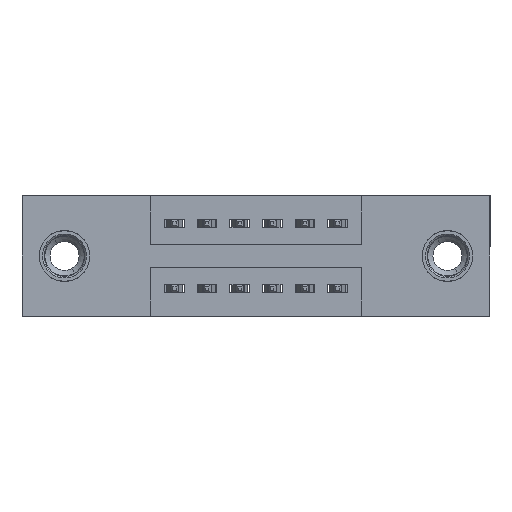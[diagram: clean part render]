
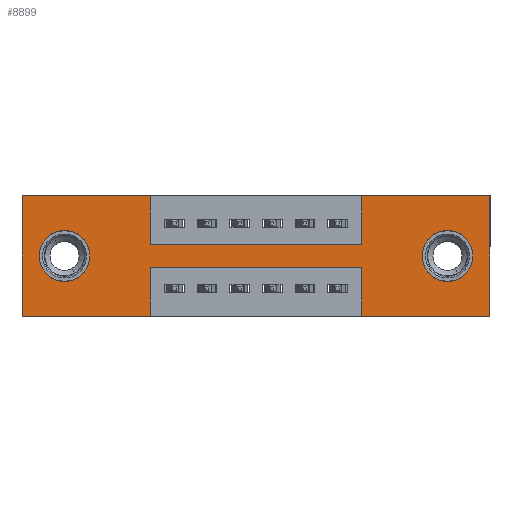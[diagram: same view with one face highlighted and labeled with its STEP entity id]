
A CAD part, front view. The second image highlights one B-rep face of the part: STEP entity #8899.
In plain terms, the highlighted planar face has unit normal (0, -1, 0).
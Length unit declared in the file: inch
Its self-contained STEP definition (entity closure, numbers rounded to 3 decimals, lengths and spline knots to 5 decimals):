
#130 = CARTESIAN_POINT ( 'NONE',  ( 0.3925, 0., -0.37 ) ) ;
#145 = VECTOR ( 'NONE', #192, 39.37008 ) ;
#192 = DIRECTION ( 'NONE',  ( -1., 0., 0. ) ) ;
#392 = AXIS2_PLACEMENT_3D ( 'NONE', #6455, #1046, #7413 ) ;
#548 = CARTESIAN_POINT ( 'NONE',  ( 1.0425, 0., -0.37 ) ) ;
#597 = EDGE_CURVE ( 'NONE', #10310, #9483, #11080, .T. ) ;
#658 = EDGE_CURVE ( 'NONE', #4016, #3449, #1130, .T. ) ;
#727 = EDGE_CURVE ( 'NONE', #2626, #7450, #7537, .T. ) ;
#729 = ORIENTED_EDGE ( 'NONE', *, *, #8642, .F. ) ;
#791 = VECTOR ( 'NONE', #1757, 39.37008 ) ;
#826 = CARTESIAN_POINT ( 'NONE',  ( 1.0425, 0., 0. ) ) ;
#850 = DIRECTION ( 'NONE',  ( 0., 0., -1. ) ) ;
#856 = VECTOR ( 'NONE', #5947, 39.37008 ) ;
#970 = CARTESIAN_POINT ( 'NONE',  ( 0.3925, 0., -0.37 ) ) ;
#1046 = DIRECTION ( 'NONE',  ( 0., 1., 0. ) ) ;
#1050 = CARTESIAN_POINT ( 'NONE',  ( 1.0425, 0., -0.22 ) ) ;
#1063 = DIRECTION ( 'NONE',  ( 0., 0., -1. ) ) ;
#1094 = ORIENTED_EDGE ( 'NONE', *, *, #5873, .T. ) ;
#1130 = LINE ( 'NONE', #11693, #856 ) ;
#1203 = ORIENTED_EDGE ( 'NONE', *, *, #6531, .F. ) ;
#1232 = CARTESIAN_POINT ( 'NONE',  ( 1.0425, 0., -0.37 ) ) ;
#1361 = CARTESIAN_POINT ( 'NONE',  ( 0., 0., -0.37 ) ) ;
#1482 = DIRECTION ( 'NONE',  ( -1., 0., 0. ) ) ;
#1496 = ORIENTED_EDGE ( 'NONE', *, *, #9762, .F. ) ;
#1508 = VERTEX_POINT ( 'NONE', #10363 ) ;
#1738 = EDGE_CURVE ( 'NONE', #7450, #7218, #3411, .T. ) ;
#1746 = CARTESIAN_POINT ( 'NONE',  ( 0.3925, 0., -0.15 ) ) ;
#1747 = VECTOR ( 'NONE', #7598, 39.37008 ) ;
#1757 = DIRECTION ( 'NONE',  ( 0., 0., 1. ) ) ;
#1804 = LINE ( 'NONE', #130, #4196 ) ;
#2055 = CARTESIAN_POINT ( 'NONE',  ( 0., 0., -0.37 ) ) ;
#2093 = VERTEX_POINT ( 'NONE', #10782 ) ;
#2450 = ORIENTED_EDGE ( 'NONE', *, *, #10242, .F. ) ;
#2568 = VECTOR ( 'NONE', #5516, 39.37008 ) ;
#2569 = CARTESIAN_POINT ( 'NONE',  ( 1.435, 0., -0.37 ) ) ;
#2626 = VERTEX_POINT ( 'NONE', #9010 ) ;
#2719 = VECTOR ( 'NONE', #6650, 39.37008 ) ;
#2881 = VERTEX_POINT ( 'NONE', #10177 ) ;
#3011 = CARTESIAN_POINT ( 'NONE',  ( 0.13, 0., -0.185 ) ) ;
#3106 = VECTOR ( 'NONE', #5590, 39.37008 ) ;
#3234 = CARTESIAN_POINT ( 'NONE',  ( 0., 0., 0. ) ) ;
#3356 = CARTESIAN_POINT ( 'NONE',  ( 0., 0., -0.37 ) ) ;
#3387 = DIRECTION ( 'NONE',  ( 0., 1., 0. ) ) ;
#3411 = LINE ( 'NONE', #5083, #2568 ) ;
#3430 = ORIENTED_EDGE ( 'NONE', *, *, #4465, .T. ) ;
#3449 = VERTEX_POINT ( 'NONE', #11041 ) ;
#3506 = LINE ( 'NONE', #3540, #5596 ) ;
#3513 = CARTESIAN_POINT ( 'NONE',  ( 0.3925, 0., 0. ) ) ;
#3540 = CARTESIAN_POINT ( 'NONE',  ( 0.3925, 0., -0.22 ) ) ;
#3805 = CARTESIAN_POINT ( 'NONE',  ( 0., 0., 0. ) ) ;
#3924 = DIRECTION ( 'NONE',  ( 0., 0., 1. ) ) ;
#3982 = LINE ( 'NONE', #4434, #5789 ) ;
#4016 = VERTEX_POINT ( 'NONE', #1746 ) ;
#4196 = VECTOR ( 'NONE', #1063, 39.37008 ) ;
#4424 = DIRECTION ( 'NONE',  ( -1., 0., 0. ) ) ;
#4434 = CARTESIAN_POINT ( 'NONE',  ( 0., 0., 0. ) ) ;
#4465 = EDGE_CURVE ( 'NONE', #1508, #2881, #6711, .T. ) ;
#4542 = LINE ( 'NONE', #5057, #4819 ) ;
#4663 = CARTESIAN_POINT ( 'NONE',  ( 1.435, 0., 0. ) ) ;
#4817 = ORIENTED_EDGE ( 'NONE', *, *, #1738, .F. ) ;
#4819 = VECTOR ( 'NONE', #1482, 39.37008 ) ;
#4836 = VERTEX_POINT ( 'NONE', #3356 ) ;
#4981 = DIRECTION ( 'NONE',  ( 0., -1., 0. ) ) ;
#5057 = CARTESIAN_POINT ( 'NONE',  ( 0., 0., -0.37 ) ) ;
#5083 = CARTESIAN_POINT ( 'NONE',  ( 1.435, 0., 0. ) ) ;
#5344 = DIRECTION ( 'NONE',  ( 1., 0., 0. ) ) ;
#5492 = LINE ( 'NONE', #3805, #3106 ) ;
#5516 = DIRECTION ( 'NONE',  ( 0., 0., -1. ) ) ;
#5581 = AXIS2_PLACEMENT_3D ( 'NONE', #10006, #3387, #9982 ) ;
#5583 = LINE ( 'NONE', #826, #791 ) ;
#5590 = DIRECTION ( 'NONE',  ( 0., 0., 1. ) ) ;
#5596 = VECTOR ( 'NONE', #4424, 39.37008 ) ;
#5616 = FACE_OUTER_BOUND ( 'NONE', #9527, .T. ) ;
#5773 = EDGE_LOOP ( 'NONE', ( #3430, #1094 ) ) ;
#5789 = VECTOR ( 'NONE', #5344, 39.37008 ) ;
#5873 = EDGE_CURVE ( 'NONE', #2881, #1508, #8297, .T. ) ;
#5947 = DIRECTION ( 'NONE',  ( 1., 0., 0. ) ) ;
#5982 = ORIENTED_EDGE ( 'NONE', *, *, #6706, .F. ) ;
#6257 = DIRECTION ( 'NONE',  ( 0., 1., 0. ) ) ;
#6293 = ORIENTED_EDGE ( 'NONE', *, *, #7260, .F. ) ;
#6330 = AXIS2_PLACEMENT_3D ( 'NONE', #1361, #4981, #11347 ) ;
#6409 = ORIENTED_EDGE ( 'NONE', *, *, #658, .F. ) ;
#6455 = CARTESIAN_POINT ( 'NONE',  ( 0.13, 0., -0.185 ) ) ;
#6466 = EDGE_CURVE ( 'NONE', #7218, #7755, #7112, .T. ) ;
#6531 = EDGE_CURVE ( 'NONE', #7755, #8623, #8989, .T. ) ;
#6650 = DIRECTION ( 'NONE',  ( 1., 0., 0. ) ) ;
#6706 = EDGE_CURVE ( 'NONE', #10977, #4836, #4542, .T. ) ;
#6711 = CIRCLE ( 'NONE', #392, 0.078 ) ;
#6933 = ORIENTED_EDGE ( 'NONE', *, *, #727, .F. ) ;
#7112 = LINE ( 'NONE', #2055, #145 ) ;
#7218 = VERTEX_POINT ( 'NONE', #2569 ) ;
#7260 = EDGE_CURVE ( 'NONE', #2093, #4016, #11213, .T. ) ;
#7277 = EDGE_CURVE ( 'NONE', #8964, #2093, #3982, .T. ) ;
#7413 = DIRECTION ( 'NONE',  ( 0., 0., 1. ) ) ;
#7418 = AXIS2_PLACEMENT_3D ( 'NONE', #3011, #9358, #3924 ) ;
#7450 = VERTEX_POINT ( 'NONE', #4663 ) ;
#7537 = LINE ( 'NONE', #3234, #2719 ) ;
#7598 = DIRECTION ( 'NONE',  ( 0., 0., 1. ) ) ;
#7755 = VERTEX_POINT ( 'NONE', #548 ) ;
#7783 = FACE_BOUND ( 'NONE', #10924, .T. ) ;
#8297 = CIRCLE ( 'NONE', #7418, 0.078 ) ;
#8449 = CIRCLE ( 'NONE', #10942, 0.078 ) ;
#8623 = VERTEX_POINT ( 'NONE', #1050 ) ;
#8642 = EDGE_CURVE ( 'NONE', #4836, #8964, #5492, .T. ) ;
#8719 = CARTESIAN_POINT ( 'NONE',  ( 0., 0., 0. ) ) ;
#8831 = VECTOR ( 'NONE', #10765, 39.37008 ) ;
#8899 = ADVANCED_FACE ( 'NONE', ( #7783, #10200, #5616 ), #10452, .T. ) ;
#8964 = VERTEX_POINT ( 'NONE', #8719 ) ;
#8989 = LINE ( 'NONE', #1232, #1747 ) ;
#9010 = CARTESIAN_POINT ( 'NONE',  ( 1.0425, 0., 0. ) ) ;
#9339 = ORIENTED_EDGE ( 'NONE', *, *, #6466, .F. ) ;
#9358 = DIRECTION ( 'NONE',  ( 0., 1., 0. ) ) ;
#9403 = ORIENTED_EDGE ( 'NONE', *, *, #9933, .F. ) ;
#9452 = VERTEX_POINT ( 'NONE', #9495 ) ;
#9468 = ORIENTED_EDGE ( 'NONE', *, *, #7277, .F. ) ;
#9483 = VERTEX_POINT ( 'NONE', #11295 ) ;
#9495 = CARTESIAN_POINT ( 'NONE',  ( 0.3925, 0., -0.22 ) ) ;
#9527 = EDGE_LOOP ( 'NONE', ( #9403, #1496, #1203, #9339, #4817, #6933, #2450, #6409, #6293, #9468, #729, #5982 ) ) ;
#9762 = EDGE_CURVE ( 'NONE', #8623, #9452, #3506, .T. ) ;
#9933 = EDGE_CURVE ( 'NONE', #9452, #10977, #1804, .T. ) ;
#9982 = DIRECTION ( 'NONE',  ( 0., 0., -1. ) ) ;
#9995 = CARTESIAN_POINT ( 'NONE',  ( 1.305, 0., -0.107 ) ) ;
#10006 = CARTESIAN_POINT ( 'NONE',  ( 1.305, 0., -0.185 ) ) ;
#10177 = CARTESIAN_POINT ( 'NONE',  ( 0.13, 0., -0.263 ) ) ;
#10200 = FACE_BOUND ( 'NONE', #5773, .T. ) ;
#10242 = EDGE_CURVE ( 'NONE', #3449, #2626, #5583, .T. ) ;
#10310 = VERTEX_POINT ( 'NONE', #9995 ) ;
#10363 = CARTESIAN_POINT ( 'NONE',  ( 0.13, 0., -0.107 ) ) ;
#10452 = PLANE ( 'NONE',  #6330 ) ;
#10496 = ORIENTED_EDGE ( 'NONE', *, *, #10893, .T. ) ;
#10765 = DIRECTION ( 'NONE',  ( 0., 0., -1. ) ) ;
#10782 = CARTESIAN_POINT ( 'NONE',  ( 0.3925, 0., 0. ) ) ;
#10889 = ORIENTED_EDGE ( 'NONE', *, *, #597, .T. ) ;
#10893 = EDGE_CURVE ( 'NONE', #9483, #10310, #8449, .T. ) ;
#10924 = EDGE_LOOP ( 'NONE', ( #10889, #10496 ) ) ;
#10942 = AXIS2_PLACEMENT_3D ( 'NONE', #11686, #6257, #850 ) ;
#10977 = VERTEX_POINT ( 'NONE', #970 ) ;
#11041 = CARTESIAN_POINT ( 'NONE',  ( 1.0425, 0., -0.15 ) ) ;
#11080 = CIRCLE ( 'NONE', #5581, 0.078 ) ;
#11213 = LINE ( 'NONE', #3513, #8831 ) ;
#11295 = CARTESIAN_POINT ( 'NONE',  ( 1.305, 0., -0.263 ) ) ;
#11347 = DIRECTION ( 'NONE',  ( 0., 0., -1. ) ) ;
#11686 = CARTESIAN_POINT ( 'NONE',  ( 1.305, 0., -0.185 ) ) ;
#11693 = CARTESIAN_POINT ( 'NONE',  ( 0.3925, 0., -0.15 ) ) ;
